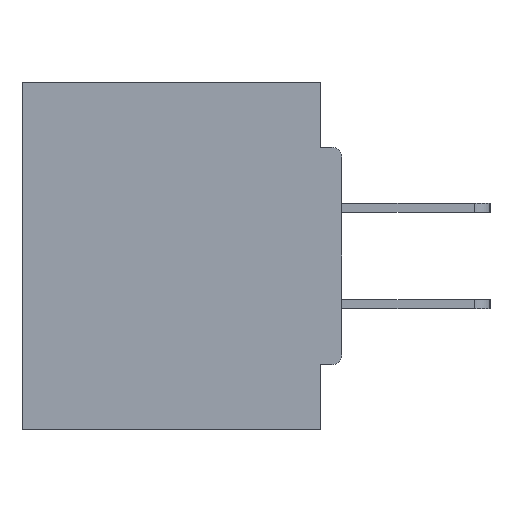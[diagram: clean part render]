
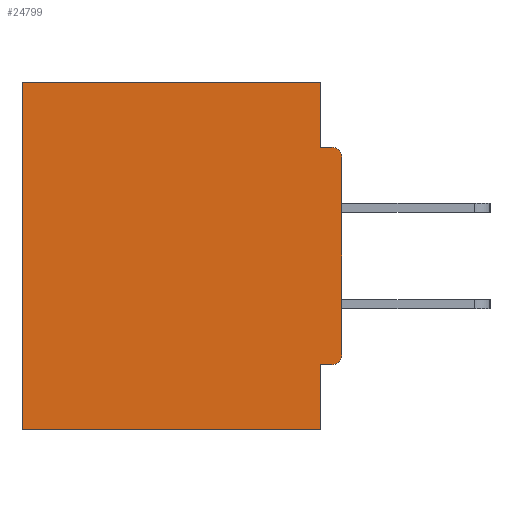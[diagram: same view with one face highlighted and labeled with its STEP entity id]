
A CAD part, left-side view. The second image highlights one B-rep face of the part: STEP entity #24799.
In plain terms, the highlighted planar face has unit normal (-1, 0, 0).
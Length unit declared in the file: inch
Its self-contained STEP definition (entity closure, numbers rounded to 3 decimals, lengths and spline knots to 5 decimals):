
#625 = DIRECTION ( 'NONE',  ( -1., 0., 0. ) ) ;
#816 = LINE ( 'NONE', #2285, #12976 ) ;
#1230 = ORIENTED_EDGE ( 'NONE', *, *, #20165, .F. ) ;
#1422 = CARTESIAN_POINT ( 'NONE',  ( 0.298, 0.031, -0.5 ) ) ;
#1483 = DIRECTION ( 'NONE',  ( 0., 1., 0. ) ) ;
#1703 = LINE ( 'NONE', #3765, #13867 ) ;
#1754 = PLANE ( 'NONE',  #8514 ) ;
#1944 = LINE ( 'NONE', #6328, #24906 ) ;
#2059 = DIRECTION ( 'NONE',  ( 0., -1., 0. ) ) ;
#2240 = ORIENTED_EDGE ( 'NONE', *, *, #22294, .T. ) ;
#2285 = CARTESIAN_POINT ( 'NONE',  ( 0.298, 0., -0.0935 ) ) ;
#2666 = CARTESIAN_POINT ( 'NONE',  ( 0.298, 0.015, -0.0935 ) ) ;
#2868 = ORIENTED_EDGE ( 'NONE', *, *, #3333, .F. ) ;
#2886 = VERTEX_POINT ( 'NONE', #9486 ) ;
#3096 = DIRECTION ( 'NONE',  ( 0., 0., -1. ) ) ;
#3333 = EDGE_CURVE ( 'NONE', #22867, #5066, #28547, .T. ) ;
#3563 = DIRECTION ( 'NONE',  ( 0., 1., 0. ) ) ;
#3765 = CARTESIAN_POINT ( 'NONE',  ( 0.298, 0., 0. ) ) ;
#3878 = CARTESIAN_POINT ( 'NONE',  ( 0.298, 0.46, -0.5 ) ) ;
#4127 = CARTESIAN_POINT ( 'NONE',  ( 0.298, 0., 0. ) ) ;
#4398 = EDGE_LOOP ( 'NONE', ( #2240, #26470, #4598, #24510, #5267, #1230, #2868, #5892, #5255, #9772 ) ) ;
#4598 = ORIENTED_EDGE ( 'NONE', *, *, #15502, .F. ) ;
#5066 = VERTEX_POINT ( 'NONE', #1422 ) ;
#5255 = ORIENTED_EDGE ( 'NONE', *, *, #7574, .T. ) ;
#5267 = ORIENTED_EDGE ( 'NONE', *, *, #5896, .T. ) ;
#5892 = ORIENTED_EDGE ( 'NONE', *, *, #25028, .F. ) ;
#5896 = EDGE_CURVE ( 'NONE', #9024, #25192, #14592, .T. ) ;
#5912 = VECTOR ( 'NONE', #3563, 39.37008 ) ;
#6328 = CARTESIAN_POINT ( 'NONE',  ( 0.298, 0., 0. ) ) ;
#6654 = VERTEX_POINT ( 'NONE', #21109 ) ;
#6867 = DIRECTION ( 'NONE',  ( 0., 0., -1. ) ) ;
#7574 = EDGE_CURVE ( 'NONE', #2886, #23039, #24488, .T. ) ;
#7580 = CIRCLE ( 'NONE', #12936, 0.015 ) ;
#7775 = DIRECTION ( 'NONE',  ( 0., 0., -1. ) ) ;
#7970 = CARTESIAN_POINT ( 'NONE',  ( 0.298, 0.46, 0. ) ) ;
#8067 = VECTOR ( 'NONE', #7775, 39.37008 ) ;
#8514 = AXIS2_PLACEMENT_3D ( 'NONE', #4127, #28589, #6867 ) ;
#9024 = VERTEX_POINT ( 'NONE', #27957 ) ;
#9304 = EDGE_CURVE ( 'NONE', #9805, #23039, #1703, .T. ) ;
#9486 = CARTESIAN_POINT ( 'NONE',  ( 0.298, 0.015, -0.4065 ) ) ;
#9772 = ORIENTED_EDGE ( 'NONE', *, *, #9304, .F. ) ;
#9805 = VERTEX_POINT ( 'NONE', #16697 ) ;
#10411 = DIRECTION ( 'NONE',  ( 0., 0., -1. ) ) ;
#12936 = AXIS2_PLACEMENT_3D ( 'NONE', #23037, #625, #3096 ) ;
#12976 = VECTOR ( 'NONE', #2059, 39.37008 ) ;
#13123 = DIRECTION ( 'NONE',  ( 0., 0., -1. ) ) ;
#13230 = LINE ( 'NONE', #24834, #19000 ) ;
#13470 = LINE ( 'NONE', #20712, #5912 ) ;
#13486 = DIRECTION ( 'NONE',  ( 0., 0., -1. ) ) ;
#13867 = VECTOR ( 'NONE', #13486, 39.37008 ) ;
#14233 = CARTESIAN_POINT ( 'NONE',  ( 0.298, 0.015, -0.3915 ) ) ;
#14592 = LINE ( 'NONE', #7970, #8067 ) ;
#15502 = EDGE_CURVE ( 'NONE', #23628, #6654, #13230, .T. ) ;
#15761 = VERTEX_POINT ( 'NONE', #2666 ) ;
#16697 = CARTESIAN_POINT ( 'NONE',  ( 0.298, 0., -0.1085 ) ) ;
#16714 = DIRECTION ( 'NONE',  ( 0., 0., -1. ) ) ;
#17424 = CARTESIAN_POINT ( 'NONE',  ( 0.298, 0.031, -0.5 ) ) ;
#17615 = CARTESIAN_POINT ( 'NONE',  ( 0.298, 0.031, 0. ) ) ;
#18367 = CARTESIAN_POINT ( 'NONE',  ( 0.298, 0.031, -0.4065 ) ) ;
#19000 = VECTOR ( 'NONE', #10411, 39.37008 ) ;
#19441 = LINE ( 'NONE', #25571, #26000 ) ;
#19523 = DIRECTION ( 'NONE',  ( -1., 0., 0. ) ) ;
#19914 = EDGE_CURVE ( 'NONE', #23628, #9024, #1944, .T. ) ;
#20165 = EDGE_CURVE ( 'NONE', #5066, #25192, #19441, .T. ) ;
#20222 = CARTESIAN_POINT ( 'NONE',  ( 0.298, 0., -0.3915 ) ) ;
#20541 = EDGE_CURVE ( 'NONE', #6654, #15761, #816, .T. ) ;
#20712 = CARTESIAN_POINT ( 'NONE',  ( 0.298, 0., -0.4065 ) ) ;
#21109 = CARTESIAN_POINT ( 'NONE',  ( 0.298, 0.031, -0.0935 ) ) ;
#22294 = EDGE_CURVE ( 'NONE', #9805, #15761, #7580, .T. ) ;
#22867 = VERTEX_POINT ( 'NONE', #18367 ) ;
#23037 = CARTESIAN_POINT ( 'NONE',  ( 0.298, 0.015, -0.1085 ) ) ;
#23039 = VERTEX_POINT ( 'NONE', #20222 ) ;
#23628 = VERTEX_POINT ( 'NONE', #17615 ) ;
#24488 = CIRCLE ( 'NONE', #30754, 0.015 ) ;
#24510 = ORIENTED_EDGE ( 'NONE', *, *, #19914, .T. ) ;
#24799 = ADVANCED_FACE ( 'NONE', ( #27363 ), #1754, .F. ) ;
#24834 = CARTESIAN_POINT ( 'NONE',  ( 0.298, 0.031, -0.5 ) ) ;
#24906 = VECTOR ( 'NONE', #31327, 39.37008 ) ;
#25028 = EDGE_CURVE ( 'NONE', #2886, #22867, #13470, .T. ) ;
#25192 = VERTEX_POINT ( 'NONE', #3878 ) ;
#25571 = CARTESIAN_POINT ( 'NONE',  ( 0.298, 0., -0.5 ) ) ;
#26000 = VECTOR ( 'NONE', #1483, 39.37008 ) ;
#26470 = ORIENTED_EDGE ( 'NONE', *, *, #20541, .F. ) ;
#27363 = FACE_OUTER_BOUND ( 'NONE', #4398, .T. ) ;
#27429 = VECTOR ( 'NONE', #13123, 39.37008 ) ;
#27957 = CARTESIAN_POINT ( 'NONE',  ( 0.298, 0.46, 0. ) ) ;
#28547 = LINE ( 'NONE', #17424, #27429 ) ;
#28589 = DIRECTION ( 'NONE',  ( 1., 0., 0. ) ) ;
#30754 = AXIS2_PLACEMENT_3D ( 'NONE', #14233, #19523, #16714 ) ;
#31327 = DIRECTION ( 'NONE',  ( 0., 1., 0. ) ) ;
